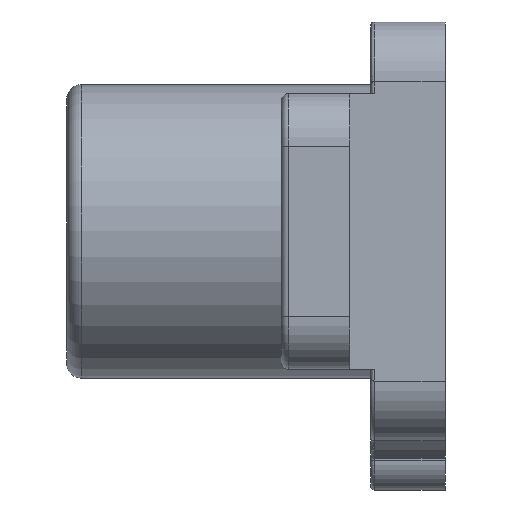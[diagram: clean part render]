
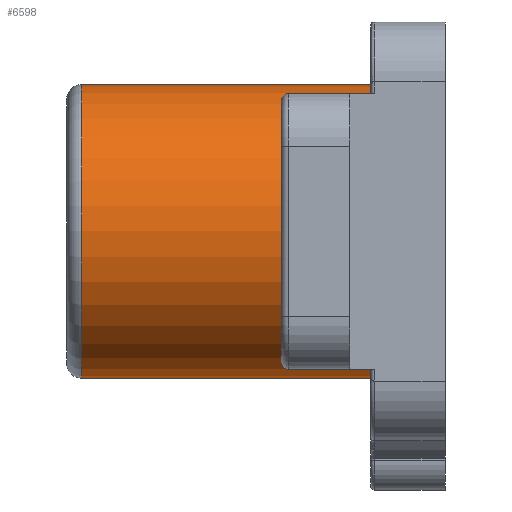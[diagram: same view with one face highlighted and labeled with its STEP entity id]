
A CAD part, front view. The second image highlights one B-rep face of the part: STEP entity #6598.
In plain terms, the highlighted cylindrical face has radius 19.709 mm (diameter 39.418 mm), a full revolution.
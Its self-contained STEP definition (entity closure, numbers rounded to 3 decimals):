
#654 = CIRCLE ( 'NONE', #1261, 19.709 ) ;
#1127 = CARTESIAN_POINT ( 'NONE',  ( -194.652, 145.704, 0. ) ) ;
#1254 = CARTESIAN_POINT ( 'NONE',  ( -227.491, 145.704, 19.709 ) ) ;
#1261 = AXIS2_PLACEMENT_3D ( 'NONE', #11691, #10758, #7705 ) ;
#2721 = VERTEX_POINT ( 'NONE', #1254 ) ;
#3143 = EDGE_LOOP ( 'NONE', ( #5804 ) ) ;
#3593 = EDGE_CURVE ( 'NONE', #6354, #6354, #654, .T. ) ;
#3658 = DIRECTION ( 'NONE',  ( 0., 0., 1. ) ) ;
#3745 = ORIENTED_EDGE ( 'NONE', *, *, #3593, .F. ) ;
#4407 = AXIS2_PLACEMENT_3D ( 'NONE', #12415, #6604, #3658 ) ;
#4735 = FACE_OUTER_BOUND ( 'NONE', #3143, .T. ) ;
#5474 = CYLINDRICAL_SURFACE ( 'NONE', #11763, 19.709 ) ;
#5804 = ORIENTED_EDGE ( 'NONE', *, *, #7595, .F. ) ;
#6354 = VERTEX_POINT ( 'NONE', #10986 ) ;
#6598 = ADVANCED_FACE ( 'NONE', ( #10620, #4735 ), #5474, .T. ) ;
#6604 = DIRECTION ( 'NONE',  ( -1., 0., 0. ) ) ;
#7595 = EDGE_CURVE ( 'NONE', #2721, #2721, #12433, .T. ) ;
#7705 = DIRECTION ( 'NONE',  ( 0., 0., 1. ) ) ;
#8318 = EDGE_LOOP ( 'NONE', ( #3745 ) ) ;
#10023 = DIRECTION ( 'NONE',  ( 0., 0., 1. ) ) ;
#10620 = FACE_OUTER_BOUND ( 'NONE', #8318, .T. ) ;
#10758 = DIRECTION ( 'NONE',  ( 1., 0., 0. ) ) ;
#10986 = CARTESIAN_POINT ( 'NONE',  ( -188.682, 145.704, 19.709 ) ) ;
#11691 = CARTESIAN_POINT ( 'NONE',  ( -188.682, 145.704, 0. ) ) ;
#11763 = AXIS2_PLACEMENT_3D ( 'NONE', #1127, #11886, #10023 ) ;
#11886 = DIRECTION ( 'NONE',  ( -1., 0., 0. ) ) ;
#12415 = CARTESIAN_POINT ( 'NONE',  ( -227.491, 145.704, 0. ) ) ;
#12433 = CIRCLE ( 'NONE', #4407, 19.709 ) ;
